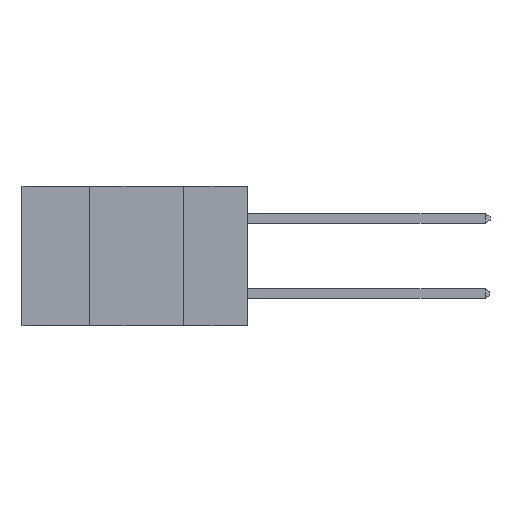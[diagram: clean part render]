
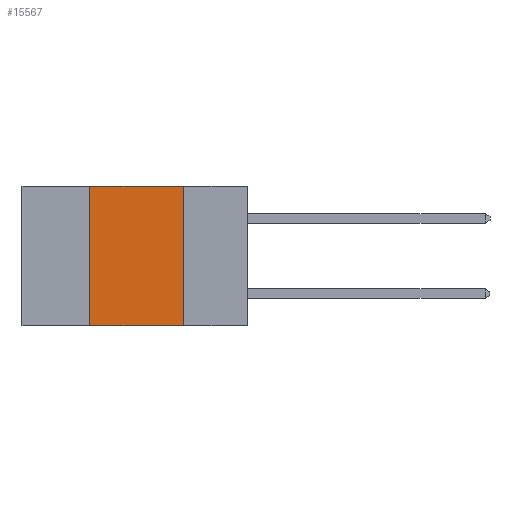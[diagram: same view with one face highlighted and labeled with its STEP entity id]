
A CAD part, left-side view. The second image highlights one B-rep face of the part: STEP entity #15567.
In plain terms, the highlighted planar face has unit normal (-1, 0, 0).
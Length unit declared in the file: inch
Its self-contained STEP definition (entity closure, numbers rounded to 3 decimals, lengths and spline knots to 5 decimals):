
#16 = VECTOR ( 'NONE', #12137, 39.37008 ) ;
#353 = CARTESIAN_POINT ( 'NONE',  ( 0., 0.17, 0. ) ) ;
#984 = DIRECTION ( 'NONE',  ( 0., -1., 0. ) ) ;
#1657 = LINE ( 'NONE', #353, #4657 ) ;
#1688 = DIRECTION ( 'NONE',  ( 0., 0., -1. ) ) ;
#1854 = EDGE_CURVE ( 'NONE', #6283, #14490, #4403, .T. ) ;
#2125 = DIRECTION ( 'NONE',  ( 1., 0., 0. ) ) ;
#2431 = ORIENTED_EDGE ( 'NONE', *, *, #4222, .T. ) ;
#2855 = CARTESIAN_POINT ( 'NONE',  ( 0., 0.42, -0.37 ) ) ;
#3184 = ORIENTED_EDGE ( 'NONE', *, *, #5043, .F. ) ;
#3741 = CARTESIAN_POINT ( 'NONE',  ( 0., 0.17, 0. ) ) ;
#4142 = FACE_OUTER_BOUND ( 'NONE', #8194, .T. ) ;
#4159 = DIRECTION ( 'NONE',  ( 0., 0., 1. ) ) ;
#4222 = EDGE_CURVE ( 'NONE', #10508, #6223, #12563, .T. ) ;
#4403 = LINE ( 'NONE', #14830, #7292 ) ;
#4657 = VECTOR ( 'NONE', #1688, 39.37008 ) ;
#5043 = EDGE_CURVE ( 'NONE', #10508, #6283, #9919, .T. ) ;
#5680 = CARTESIAN_POINT ( 'NONE',  ( 0., 0.42, 0. ) ) ;
#5883 = EDGE_CURVE ( 'NONE', #14490, #6223, #1657, .T. ) ;
#6083 = CARTESIAN_POINT ( 'NONE',  ( 0., 0.6, -0.37 ) ) ;
#6136 = CARTESIAN_POINT ( 'NONE',  ( 0., 0.42, 0. ) ) ;
#6223 = VERTEX_POINT ( 'NONE', #13317 ) ;
#6283 = VERTEX_POINT ( 'NONE', #6136 ) ;
#6588 = VECTOR ( 'NONE', #4159, 39.37008 ) ;
#7292 = VECTOR ( 'NONE', #984, 39.37008 ) ;
#8194 = EDGE_LOOP ( 'NONE', ( #8737, #8452, #3184, #2431 ) ) ;
#8360 = PLANE ( 'NONE',  #15529 ) ;
#8452 = ORIENTED_EDGE ( 'NONE', *, *, #1854, .F. ) ;
#8737 = ORIENTED_EDGE ( 'NONE', *, *, #5883, .F. ) ;
#9636 = CARTESIAN_POINT ( 'NONE',  ( 0., 0.6, 0. ) ) ;
#9919 = LINE ( 'NONE', #5680, #6588 ) ;
#10508 = VERTEX_POINT ( 'NONE', #2855 ) ;
#10886 = DIRECTION ( 'NONE',  ( 0., 0., -1. ) ) ;
#12137 = DIRECTION ( 'NONE',  ( 0., -1., 0. ) ) ;
#12563 = LINE ( 'NONE', #6083, #16 ) ;
#13317 = CARTESIAN_POINT ( 'NONE',  ( 0., 0.17, -0.37 ) ) ;
#14490 = VERTEX_POINT ( 'NONE', #3741 ) ;
#14830 = CARTESIAN_POINT ( 'NONE',  ( 0., 0.6, 0. ) ) ;
#15529 = AXIS2_PLACEMENT_3D ( 'NONE', #9636, #2125, #10886 ) ;
#15567 = ADVANCED_FACE ( 'NONE', ( #4142 ), #8360, .F. ) ;
